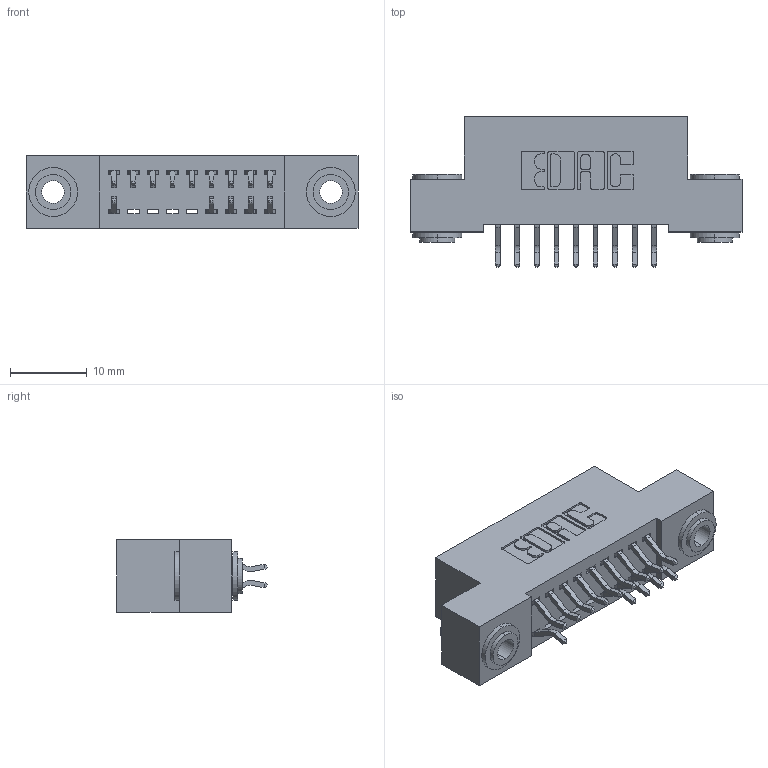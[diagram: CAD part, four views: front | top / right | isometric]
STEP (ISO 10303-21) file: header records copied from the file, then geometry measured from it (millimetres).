
FILE_DESCRIPTION (( 'STEP AP203' ), '1' );
FILE_NAME ('392-018-556-203.STEP', '2018-08-15T04:40:59', ( '' ), ( '' ), 'SwSTEP 2.0', 'SolidWorks 2016', '' );
FILE_SCHEMA (( 'CONFIG_CONTROL_DESIGN' ));
Length unit declared in the file: inch
Products named in the file (4): 345-292-001_556 Tail; 342-250-002_345-250-002-102; 392-018-556-203; 342 Part_.156 TH
Assembly tree (17 placements, depth 2):
  392-018-556-203
    342 Part_.156 TH
    345-292-001_556 Tail  x14
    342-250-002_345-250-002-102  x2
Bounding box: 43.18 x 19.58 x 9.4 mm (x, y, z)
Volume: 3710 mm3; surface area: 5227.3 mm2
Topology: 17 solids, 17 shells, 984 faces, 2881 edges, 1898 vertices
Faces by surface type: plane 660, cylinder 316, cone 8
Entity records: 10668 total; most frequent: CARTESIAN_POINT 1813, ORIENTED_EDGE 1734, DIRECTION 1625, EDGE_CURVE 867, VECTOR 707, LINE 707, VERTEX_POINT 574, AXIS2_PLACEMENT_3D 459
